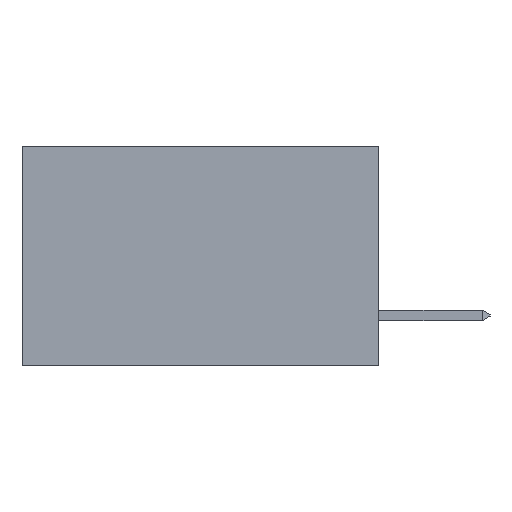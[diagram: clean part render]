
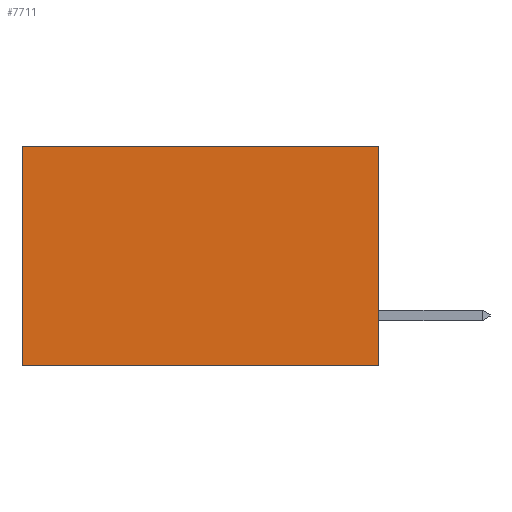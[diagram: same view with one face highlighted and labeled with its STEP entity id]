
A CAD part, left-side view. The second image highlights one B-rep face of the part: STEP entity #7711.
In plain terms, the highlighted planar face has unit normal (-1, 0, 0).
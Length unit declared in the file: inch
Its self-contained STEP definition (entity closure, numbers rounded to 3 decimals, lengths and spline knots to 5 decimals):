
#976 = VECTOR ( 'NONE', #22691, 39.37008 ) ;
#1205 = VECTOR ( 'NONE', #10081, 39.37008 ) ;
#1342 = VECTOR ( 'NONE', #16537, 39.37008 ) ;
#1495 = VERTEX_POINT ( 'NONE', #4228 ) ;
#1835 = DIRECTION ( 'NONE',  ( 1., 0., 0. ) ) ;
#2469 = CARTESIAN_POINT ( 'NONE',  ( 0.2615, 0.6, -0.37 ) ) ;
#3746 = ORIENTED_EDGE ( 'NONE', *, *, #15990, .F. ) ;
#4228 = CARTESIAN_POINT ( 'NONE',  ( 0.2615, 0., -0.37 ) ) ;
#5651 = CARTESIAN_POINT ( 'NONE',  ( 0.2615, 0.6, 0. ) ) ;
#6022 = CARTESIAN_POINT ( 'NONE',  ( 0.2615, 0., 0. ) ) ;
#6400 = LINE ( 'NONE', #18575, #976 ) ;
#7061 = EDGE_LOOP ( 'NONE', ( #17527, #25575, #3746, #17190 ) ) ;
#7711 = ADVANCED_FACE ( 'NONE', ( #23793 ), #21829, .F. ) ;
#7780 = EDGE_CURVE ( 'NONE', #17011, #20540, #12011, .T. ) ;
#9672 = LINE ( 'NONE', #15118, #14368 ) ;
#10081 = DIRECTION ( 'NONE',  ( 0., 1., 0. ) ) ;
#11438 = EDGE_CURVE ( 'NONE', #20540, #14280, #11520, .T. ) ;
#11520 = LINE ( 'NONE', #2469, #1342 ) ;
#12011 = LINE ( 'NONE', #6022, #1205 ) ;
#12082 = EDGE_CURVE ( 'NONE', #1495, #14280, #6400, .T. ) ;
#13855 = CARTESIAN_POINT ( 'NONE',  ( 0.2615, 0.6, -0.37 ) ) ;
#14280 = VERTEX_POINT ( 'NONE', #13855 ) ;
#14368 = VECTOR ( 'NONE', #19095, 39.37008 ) ;
#15118 = CARTESIAN_POINT ( 'NONE',  ( 0.2615, 0., -0.37 ) ) ;
#15911 = DIRECTION ( 'NONE',  ( 0., 0., -1. ) ) ;
#15990 = EDGE_CURVE ( 'NONE', #17011, #1495, #9672, .T. ) ;
#16537 = DIRECTION ( 'NONE',  ( 0., 0., -1. ) ) ;
#17011 = VERTEX_POINT ( 'NONE', #18527 ) ;
#17190 = ORIENTED_EDGE ( 'NONE', *, *, #7780, .T. ) ;
#17527 = ORIENTED_EDGE ( 'NONE', *, *, #11438, .T. ) ;
#18527 = CARTESIAN_POINT ( 'NONE',  ( 0.2615, 0., 0. ) ) ;
#18575 = CARTESIAN_POINT ( 'NONE',  ( 0.2615, 0., -0.37 ) ) ;
#19095 = DIRECTION ( 'NONE',  ( 0., 0., -1. ) ) ;
#20540 = VERTEX_POINT ( 'NONE', #5651 ) ;
#21829 = PLANE ( 'NONE',  #23530 ) ;
#22691 = DIRECTION ( 'NONE',  ( 0., 1., 0. ) ) ;
#23530 = AXIS2_PLACEMENT_3D ( 'NONE', #25807, #1835, #15911 ) ;
#23793 = FACE_OUTER_BOUND ( 'NONE', #7061, .T. ) ;
#25575 = ORIENTED_EDGE ( 'NONE', *, *, #12082, .F. ) ;
#25807 = CARTESIAN_POINT ( 'NONE',  ( 0.2615, 0., -0.37 ) ) ;
